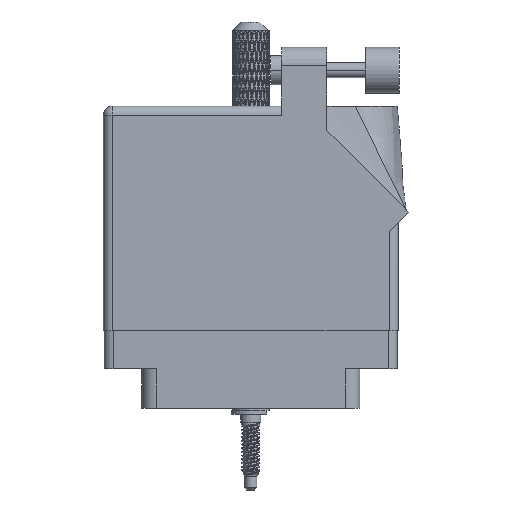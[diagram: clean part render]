
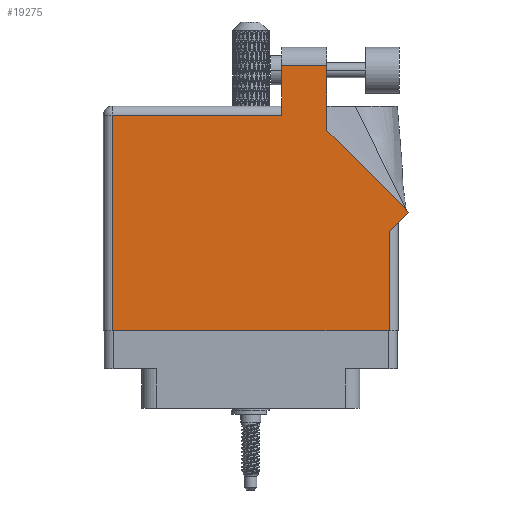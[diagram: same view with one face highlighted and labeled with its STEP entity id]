
A CAD part, front view. The second image highlights one B-rep face of the part: STEP entity #19275.
In plain terms, the highlighted face is planar.
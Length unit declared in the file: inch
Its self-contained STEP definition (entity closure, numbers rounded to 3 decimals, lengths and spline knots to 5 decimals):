
#2616 = LINE ( 'NONE', #54142, #12699 ) ;
#5091 = DIRECTION ( 'NONE',  ( 0., 1., 0. ) ) ;
#6064 = ORIENTED_EDGE ( 'NONE', *, *, #61525, .T. ) ;
#6159 = ORIENTED_EDGE ( 'NONE', *, *, #98116, .T. ) ;
#8196 = CARTESIAN_POINT ( 'NONE',  ( 0.062, 0., 0. ) ) ;
#8255 = CARTESIAN_POINT ( 'NONE',  ( 0., 0., 0. ) ) ;
#8345 = VERTEX_POINT ( 'NONE', #73245 ) ;
#9634 = DIRECTION ( 'NONE',  ( 0., -1., 0. ) ) ;
#9979 = VECTOR ( 'NONE', #32547, 39.37008 ) ;
#12699 = VECTOR ( 'NONE', #5091, 39.37008 ) ;
#15183 = VERTEX_POINT ( 'NONE', #65434 ) ;
#15607 = CARTESIAN_POINT ( 'NONE',  ( 1.524, 1.36442, 0. ) ) ;
#16731 = CARTESIAN_POINT ( 'NONE',  ( 1.948, 0., 0. ) ) ;
#19275 = ADVANCED_FACE ( 'NONE', ( #61233 ), #25909, .F. ) ;
#19519 = EDGE_CURVE ( 'NONE', #8345, #88712, #30736, .T. ) ;
#20572 = CARTESIAN_POINT ( 'NONE',  ( 2.01, 0.737, 0. ) ) ;
#22132 = LINE ( 'NONE', #50212, #71544 ) ;
#25705 = VERTEX_POINT ( 'NONE', #16731 ) ;
#25909 = PLANE ( 'NONE',  #88590 ) ;
#26258 = DIRECTION ( 'NONE',  ( 0., 0., -1. ) ) ;
#28043 = EDGE_CURVE ( 'NONE', #59040, #15183, #68893, .T. ) ;
#29162 = VERTEX_POINT ( 'NONE', #77237 ) ;
#30736 = LINE ( 'NONE', #62714, #84015 ) ;
#32547 = DIRECTION ( 'NONE',  ( 1., 0., 0. ) ) ;
#36262 = EDGE_CURVE ( 'NONE', #88712, #29162, #22132, .T. ) ;
#38928 = DIRECTION ( 'NONE',  ( 0., -1., 0. ) ) ;
#40513 = LINE ( 'NONE', #15607, #67175 ) ;
#42144 = ORIENTED_EDGE ( 'NONE', *, *, #55310, .T. ) ;
#44842 = ORIENTED_EDGE ( 'NONE', *, *, #86873, .T. ) ;
#45026 = DIRECTION ( 'NONE',  ( -1., 0., 0. ) ) ;
#46624 = LINE ( 'NONE', #8255, #9979 ) ;
#47784 = EDGE_LOOP ( 'NONE', ( #6159, #42144, #76649, #66103, #44842, #71449, #6064, #55949, #71655 ) ) ;
#48861 = DIRECTION ( 'NONE',  ( -0.707, 0.707, 0. ) ) ;
#50212 = CARTESIAN_POINT ( 'NONE',  ( 0., 1.468, 0. ) ) ;
#51109 = VECTOR ( 'NONE', #101196, 39.37008 ) ;
#54142 = CARTESIAN_POINT ( 'NONE',  ( 1.948, 0.737, 0. ) ) ;
#54191 = CARTESIAN_POINT ( 'NONE',  ( 1.217, 1.805, 0. ) ) ;
#55310 = EDGE_CURVE ( 'NONE', #104368, #8345, #69216, .T. ) ;
#55949 = ORIENTED_EDGE ( 'NONE', *, *, #28043, .T. ) ;
#56252 = DIRECTION ( 'NONE',  ( 0., 1., 0. ) ) ;
#59040 = VERTEX_POINT ( 'NONE', #66610 ) ;
#61233 = FACE_OUTER_BOUND ( 'NONE', #47784, .T. ) ;
#61525 = EDGE_CURVE ( 'NONE', #25705, #59040, #2616, .T. ) ;
#62714 = CARTESIAN_POINT ( 'NONE',  ( 1.217, 1.53, 0. ) ) ;
#65434 = CARTESIAN_POINT ( 'NONE',  ( 2.08071, 0.80771, 0. ) ) ;
#66103 = ORIENTED_EDGE ( 'NONE', *, *, #36262, .T. ) ;
#66610 = CARTESIAN_POINT ( 'NONE',  ( 1.948, 0.675, 0. ) ) ;
#66867 = LINE ( 'NONE', #90290, #71977 ) ;
#67175 = VECTOR ( 'NONE', #56252, 39.37008 ) ;
#68893 = LINE ( 'NONE', #20572, #51109 ) ;
#69216 = LINE ( 'NONE', #54191, #104572 ) ;
#71449 = ORIENTED_EDGE ( 'NONE', *, *, #86882, .T. ) ;
#71544 = VECTOR ( 'NONE', #83513, 39.37008 ) ;
#71655 = ORIENTED_EDGE ( 'NONE', *, *, #86519, .T. ) ;
#71977 = VECTOR ( 'NONE', #9634, 39.37008 ) ;
#73245 = CARTESIAN_POINT ( 'NONE',  ( 1.217, 1.805, 0. ) ) ;
#74535 = CARTESIAN_POINT ( 'NONE',  ( 1.524, 1.36442, 0. ) ) ;
#75031 = CARTESIAN_POINT ( 'NONE',  ( 1.217, 1.468, 0. ) ) ;
#75448 = VERTEX_POINT ( 'NONE', #8196 ) ;
#76649 = ORIENTED_EDGE ( 'NONE', *, *, #19519, .T. ) ;
#77237 = CARTESIAN_POINT ( 'NONE',  ( 0.062, 1.468, 0. ) ) ;
#81175 = CARTESIAN_POINT ( 'NONE',  ( 2.08071, 0.80771, 0. ) ) ;
#82596 = CARTESIAN_POINT ( 'NONE',  ( 0., 1.53, 0. ) ) ;
#82932 = DIRECTION ( 'NONE',  ( -1., 0., 0. ) ) ;
#83051 = VERTEX_POINT ( 'NONE', #74535 ) ;
#83513 = DIRECTION ( 'NONE',  ( -1., 0., 0. ) ) ;
#84015 = VECTOR ( 'NONE', #38928, 39.37008 ) ;
#86519 = EDGE_CURVE ( 'NONE', #15183, #83051, #98608, .T. ) ;
#86873 = EDGE_CURVE ( 'NONE', #29162, #75448, #66867, .T. ) ;
#86882 = EDGE_CURVE ( 'NONE', #75448, #25705, #46624, .T. ) ;
#88590 = AXIS2_PLACEMENT_3D ( 'NONE', #82596, #26258, #82932 ) ;
#88712 = VERTEX_POINT ( 'NONE', #75031 ) ;
#90290 = CARTESIAN_POINT ( 'NONE',  ( 0.062, 0., 0. ) ) ;
#92309 = CARTESIAN_POINT ( 'NONE',  ( 1.524, 1.805, 0. ) ) ;
#96055 = VECTOR ( 'NONE', #48861, 39.37008 ) ;
#98116 = EDGE_CURVE ( 'NONE', #83051, #104368, #40513, .T. ) ;
#98608 = LINE ( 'NONE', #81175, #96055 ) ;
#101196 = DIRECTION ( 'NONE',  ( 0.707, 0.707, 0. ) ) ;
#104368 = VERTEX_POINT ( 'NONE', #92309 ) ;
#104572 = VECTOR ( 'NONE', #45026, 39.37008 ) ;
